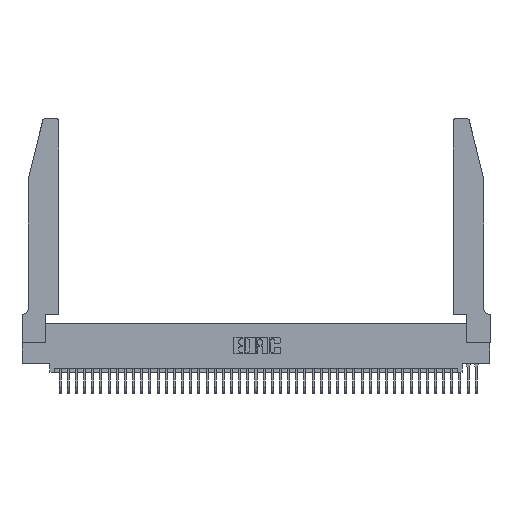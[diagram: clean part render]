
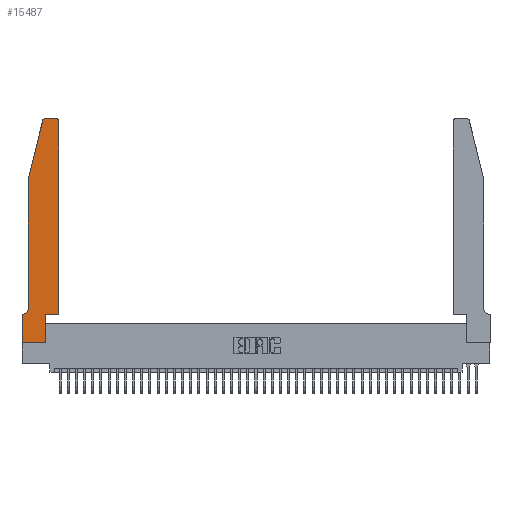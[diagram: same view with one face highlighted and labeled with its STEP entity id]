
A CAD part, top view. The second image highlights one B-rep face of the part: STEP entity #15487.
In plain terms, the highlighted planar face has unit normal (0, 0, 1).
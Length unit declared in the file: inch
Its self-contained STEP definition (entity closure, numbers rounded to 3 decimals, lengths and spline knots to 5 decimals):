
#456 = CARTESIAN_POINT ( 'NONE',  ( 0.0055, 0.42, 0.37 ) ) ;
#671 = EDGE_LOOP ( 'NONE', ( #38161, #9075, #13117, #26188, #3845, #13823, #2664, #25027, #28121, #29767, #10246, #39213 ) ) ;
#1239 = CARTESIAN_POINT ( 'NONE',  ( 0.4505, 0.35, 0.37 ) ) ;
#1752 = EDGE_CURVE ( 'NONE', #31652, #18764, #4285, .T. ) ;
#1960 = CARTESIAN_POINT ( 'NONE',  ( 0.284, 2.72, 0.37 ) ) ;
#2472 = VERTEX_POINT ( 'NONE', #24886 ) ;
#2664 = ORIENTED_EDGE ( 'NONE', *, *, #1752, .T. ) ;
#2712 = LINE ( 'NONE', #9905, #35436 ) ;
#3042 = EDGE_CURVE ( 'NONE', #8731, #14076, #3822, .T. ) ;
#3191 = VECTOR ( 'NONE', #32936, 39.37008 ) ;
#3279 = CARTESIAN_POINT ( 'NONE',  ( 0., 0.35, 0.37 ) ) ;
#3542 = CARTESIAN_POINT ( 'NONE',  ( 0.2865, 0.35, 0.37 ) ) ;
#3727 = DIRECTION ( 'NONE',  ( -1., 0., 0. ) ) ;
#3822 = LINE ( 'NONE', #12124, #19930 ) ;
#3845 = ORIENTED_EDGE ( 'NONE', *, *, #23594, .T. ) ;
#4285 = LINE ( 'NONE', #30927, #28676 ) ;
#4392 = EDGE_CURVE ( 'NONE', #14076, #19171, #19817, .T. ) ;
#5211 = DIRECTION ( 'NONE',  ( 1., 0., 0. ) ) ;
#5555 = CARTESIAN_POINT ( 'NONE',  ( 0.4505, 2.72, 0.37 ) ) ;
#5685 = DIRECTION ( 'NONE',  ( 0., -1., 0. ) ) ;
#6034 = CARTESIAN_POINT ( 'NONE',  ( 0.2605, 2.75, 0.37 ) ) ;
#6986 = PLANE ( 'NONE',  #15596 ) ;
#8731 = VERTEX_POINT ( 'NONE', #34679 ) ;
#8823 = DIRECTION ( 'NONE',  ( 0., -1., 0. ) ) ;
#9075 = ORIENTED_EDGE ( 'NONE', *, *, #22584, .T. ) ;
#9723 = CIRCLE ( 'NONE', #37556, 0.03 ) ;
#9905 = CARTESIAN_POINT ( 'NONE',  ( 0.4505, 0.35, 0.37 ) ) ;
#10192 = VERTEX_POINT ( 'NONE', #10675 ) ;
#10246 = ORIENTED_EDGE ( 'NONE', *, *, #13923, .T. ) ;
#10286 = DIRECTION ( 'NONE',  ( 0., 0., 1. ) ) ;
#10337 = VECTOR ( 'NONE', #5685, 39.37008 ) ;
#10675 = CARTESIAN_POINT ( 'NONE',  ( 0.0055, 0.35, 0.37 ) ) ;
#11207 = CARTESIAN_POINT ( 'NONE',  ( 0.0755, 0.42, 0.37 ) ) ;
#12124 = CARTESIAN_POINT ( 'NONE',  ( 0.0755, 2., 0.37 ) ) ;
#12283 = CARTESIAN_POINT ( 'NONE',  ( 0.4505, 0.35, 0.37 ) ) ;
#13117 = ORIENTED_EDGE ( 'NONE', *, *, #3042, .T. ) ;
#13133 = DIRECTION ( 'NONE',  ( 0., 1., 0. ) ) ;
#13331 = EDGE_CURVE ( 'NONE', #10192, #31652, #34992, .T. ) ;
#13823 = ORIENTED_EDGE ( 'NONE', *, *, #13331, .T. ) ;
#13923 = EDGE_CURVE ( 'NONE', #36724, #35368, #2712, .T. ) ;
#14076 = VERTEX_POINT ( 'NONE', #17078 ) ;
#15337 = DIRECTION ( 'NONE',  ( -0.239, -0.971, 0. ) ) ;
#15447 = VERTEX_POINT ( 'NONE', #16597 ) ;
#15487 = ADVANCED_FACE ( 'NONE', ( #23642 ), #6986, .T. ) ;
#15596 = AXIS2_PLACEMENT_3D ( 'NONE', #29177, #10286, #32332 ) ;
#16036 = DIRECTION ( 'NONE',  ( 0., 0., 1. ) ) ;
#16597 = CARTESIAN_POINT ( 'NONE',  ( 0.284, 2.75, 0.37 ) ) ;
#17078 = CARTESIAN_POINT ( 'NONE',  ( 0.0755, 2., 0.37 ) ) ;
#17736 = EDGE_CURVE ( 'NONE', #2472, #19004, #40936, .T. ) ;
#18764 = VERTEX_POINT ( 'NONE', #21654 ) ;
#19004 = VERTEX_POINT ( 'NONE', #29265 ) ;
#19171 = VERTEX_POINT ( 'NONE', #11207 ) ;
#19817 = LINE ( 'NONE', #21666, #10337 ) ;
#19930 = VECTOR ( 'NONE', #15337, 39.37008 ) ;
#20997 = EDGE_CURVE ( 'NONE', #23111, #15447, #31502, .T. ) ;
#21654 = CARTESIAN_POINT ( 'NONE',  ( 0., 0., 0.37 ) ) ;
#21666 = CARTESIAN_POINT ( 'NONE',  ( 0.0755, 2., 0.37 ) ) ;
#21957 = DIRECTION ( 'NONE',  ( 1., 0., 0. ) ) ;
#22584 = EDGE_CURVE ( 'NONE', #15447, #8731, #26275, .T. ) ;
#22931 = AXIS2_PLACEMENT_3D ( 'NONE', #456, #22940, #3727 ) ;
#22940 = DIRECTION ( 'NONE',  ( 0., 0., -1. ) ) ;
#23111 = VERTEX_POINT ( 'NONE', #29764 ) ;
#23565 = VECTOR ( 'NONE', #21957, 39.37008 ) ;
#23594 = EDGE_CURVE ( 'NONE', #19171, #10192, #27655, .T. ) ;
#23642 = FACE_OUTER_BOUND ( 'NONE', #671, .T. ) ;
#24362 = DIRECTION ( 'NONE',  ( 0., 0., 1. ) ) ;
#24740 = EDGE_CURVE ( 'NONE', #19004, #36724, #28594, .T. ) ;
#24886 = CARTESIAN_POINT ( 'NONE',  ( 0.2865, 0., 0.37 ) ) ;
#25027 = ORIENTED_EDGE ( 'NONE', *, *, #26567, .T. ) ;
#25290 = DIRECTION ( 'NONE',  ( -1., 0., 0. ) ) ;
#25409 = VECTOR ( 'NONE', #28993, 39.37008 ) ;
#25671 = EDGE_CURVE ( 'NONE', #35368, #23111, #9723, .T. ) ;
#26188 = ORIENTED_EDGE ( 'NONE', *, *, #4392, .T. ) ;
#26275 = CIRCLE ( 'NONE', #39815, 0.03 ) ;
#26567 = EDGE_CURVE ( 'NONE', #18764, #2472, #31837, .T. ) ;
#27655 = CIRCLE ( 'NONE', #22931, 0.07 ) ;
#28121 = ORIENTED_EDGE ( 'NONE', *, *, #17736, .T. ) ;
#28594 = LINE ( 'NONE', #1239, #3191 ) ;
#28676 = VECTOR ( 'NONE', #8823, 39.37008 ) ;
#28993 = DIRECTION ( 'NONE',  ( 0., 1., 0. ) ) ;
#29177 = CARTESIAN_POINT ( 'NONE',  ( 0., 0.35, 0.37 ) ) ;
#29265 = CARTESIAN_POINT ( 'NONE',  ( 0.2865, 0.35, 0.37 ) ) ;
#29764 = CARTESIAN_POINT ( 'NONE',  ( 0.4205, 2.75, 0.37 ) ) ;
#29767 = ORIENTED_EDGE ( 'NONE', *, *, #24740, .T. ) ;
#30530 = VECTOR ( 'NONE', #25290, 39.37008 ) ;
#30927 = CARTESIAN_POINT ( 'NONE',  ( 0., 0., 0.37 ) ) ;
#31502 = LINE ( 'NONE', #6034, #30530 ) ;
#31652 = VERTEX_POINT ( 'NONE', #3279 ) ;
#31837 = LINE ( 'NONE', #37439, #23565 ) ;
#32153 = CARTESIAN_POINT ( 'NONE',  ( 0.0755, 0.35, 0.37 ) ) ;
#32332 = DIRECTION ( 'NONE',  ( 1., 0., 0. ) ) ;
#32936 = DIRECTION ( 'NONE',  ( 1., 0., 0. ) ) ;
#34039 = VECTOR ( 'NONE', #35261, 39.37008 ) ;
#34679 = CARTESIAN_POINT ( 'NONE',  ( 0.25487, 2.72718, 0.37 ) ) ;
#34758 = CARTESIAN_POINT ( 'NONE',  ( 0.4205, 2.72, 0.37 ) ) ;
#34992 = LINE ( 'NONE', #32153, #34039 ) ;
#35261 = DIRECTION ( 'NONE',  ( -1., 0., 0. ) ) ;
#35368 = VERTEX_POINT ( 'NONE', #5555 ) ;
#35436 = VECTOR ( 'NONE', #13133, 39.37008 ) ;
#36724 = VERTEX_POINT ( 'NONE', #12283 ) ;
#37439 = CARTESIAN_POINT ( 'NONE',  ( 0., 0., 0.37 ) ) ;
#37556 = AXIS2_PLACEMENT_3D ( 'NONE', #34758, #16036, #37869 ) ;
#37869 = DIRECTION ( 'NONE',  ( 1., 0., 0. ) ) ;
#38161 = ORIENTED_EDGE ( 'NONE', *, *, #20997, .T. ) ;
#39213 = ORIENTED_EDGE ( 'NONE', *, *, #25671, .T. ) ;
#39815 = AXIS2_PLACEMENT_3D ( 'NONE', #1960, #24362, #5211 ) ;
#40936 = LINE ( 'NONE', #3542, #25409 ) ;
